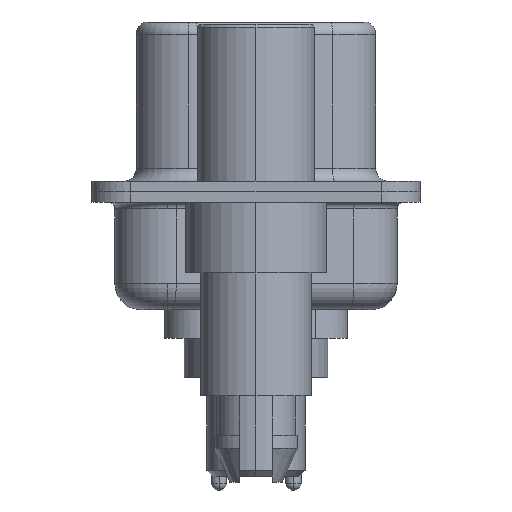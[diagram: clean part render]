
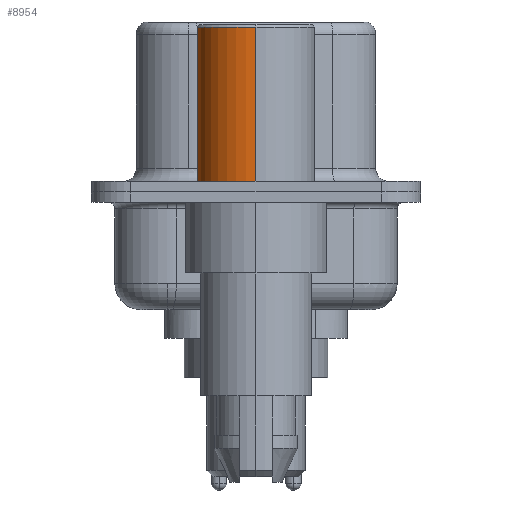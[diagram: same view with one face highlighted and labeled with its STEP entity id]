
A CAD part, left-side view. The second image highlights one B-rep face of the part: STEP entity #8954.
In plain terms, the highlighted cylindrical face has radius 2.25 mm (diameter 4.5 mm), a partial arc.
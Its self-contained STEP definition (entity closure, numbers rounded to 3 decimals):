
#544 = VERTEX_POINT ( 'NONE', #9342 ) ;
#1036 = VERTEX_POINT ( 'NONE', #2836 ) ;
#1809 = DIRECTION ( 'NONE',  ( 0., 0., 1. ) ) ;
#2392 = CARTESIAN_POINT ( 'NONE',  ( 0., 0., 0.581 ) ) ;
#2836 = CARTESIAN_POINT ( 'NONE',  ( -2.25, 0., 0.4 ) ) ;
#3455 = CIRCLE ( 'NONE', #9670, 2.25 ) ;
#4858 = ORIENTED_EDGE ( 'NONE', *, *, #18243, .F. ) ;
#6818 = EDGE_CURVE ( 'NONE', #1036, #544, #15744, .T. ) ;
#6842 = EDGE_CURVE ( 'NONE', #11697, #1036, #15323, .T. ) ;
#6998 = EDGE_CURVE ( 'NONE', #14737, #544, #3455, .T. ) ;
#7099 = DIRECTION ( 'NONE',  ( 0., 0., 1. ) ) ;
#7144 = CARTESIAN_POINT ( 'NONE',  ( -2.25, 0., 0.581 ) ) ;
#7891 = VECTOR ( 'NONE', #13282, 1000. ) ;
#8012 = ORIENTED_EDGE ( 'NONE', *, *, #6818, .T. ) ;
#8087 = ORIENTED_EDGE ( 'NONE', *, *, #6998, .F. ) ;
#8632 = VECTOR ( 'NONE', #15034, 1000. ) ;
#8709 = DIRECTION ( 'NONE',  ( 1., 0., 0. ) ) ;
#8954 = ADVANCED_FACE ( 'NONE', ( #17866 ), #13731, .T. ) ;
#8994 = DIRECTION ( 'NONE',  ( 0., 0., 1. ) ) ;
#9342 = CARTESIAN_POINT ( 'NONE',  ( -2.25, 0., 6.3 ) ) ;
#9670 = AXIS2_PLACEMENT_3D ( 'NONE', #11144, #1809, #12608 ) ;
#10069 = AXIS2_PLACEMENT_3D ( 'NONE', #17591, #8994, #19022 ) ;
#10168 = ORIENTED_EDGE ( 'NONE', *, *, #6842, .T. ) ;
#11144 = CARTESIAN_POINT ( 'NONE',  ( 0., 0., 6.3 ) ) ;
#11697 = VERTEX_POINT ( 'NONE', #18768 ) ;
#12490 = EDGE_LOOP ( 'NONE', ( #10168, #8012, #8087, #4858 ) ) ;
#12608 = DIRECTION ( 'NONE',  ( 1., 0., 0. ) ) ;
#13282 = DIRECTION ( 'NONE',  ( 0., 0., 1. ) ) ;
#13700 = CARTESIAN_POINT ( 'NONE',  ( 2.25, 0., 0.581 ) ) ;
#13731 = CYLINDRICAL_SURFACE ( 'NONE', #16107, 2.25 ) ;
#14737 = VERTEX_POINT ( 'NONE', #16820 ) ;
#15034 = DIRECTION ( 'NONE',  ( 0., 0., 1. ) ) ;
#15323 = CIRCLE ( 'NONE', #10069, 2.25 ) ;
#15744 = LINE ( 'NONE', #7144, #7891 ) ;
#15946 = LINE ( 'NONE', #13700, #8632 ) ;
#16107 = AXIS2_PLACEMENT_3D ( 'NONE', #2392, #7099, #8709 ) ;
#16820 = CARTESIAN_POINT ( 'NONE',  ( 2.25, 0., 6.3 ) ) ;
#17591 = CARTESIAN_POINT ( 'NONE',  ( 0., 0., 0.4 ) ) ;
#17866 = FACE_OUTER_BOUND ( 'NONE', #12490, .T. ) ;
#18243 = EDGE_CURVE ( 'NONE', #11697, #14737, #15946, .T. ) ;
#18768 = CARTESIAN_POINT ( 'NONE',  ( 2.25, 0., 0.4 ) ) ;
#19022 = DIRECTION ( 'NONE',  ( 1., 0., 0. ) ) ;
